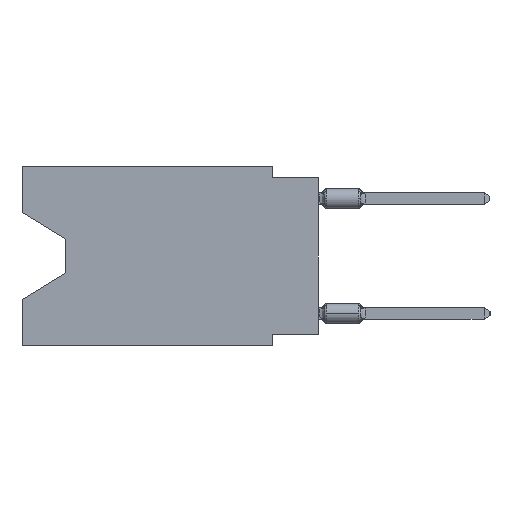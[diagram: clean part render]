
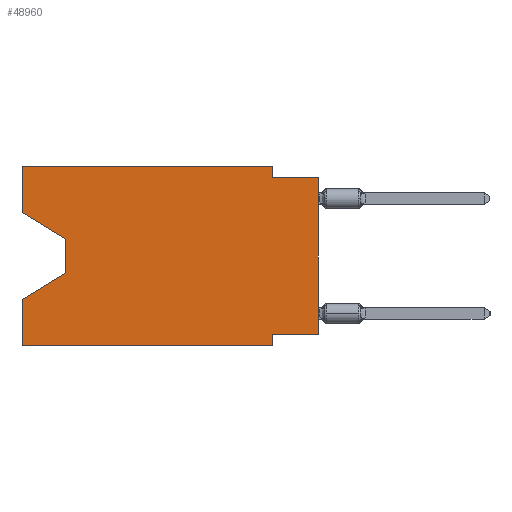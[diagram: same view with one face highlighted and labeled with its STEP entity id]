
A CAD part, left-side view. The second image highlights one B-rep face of the part: STEP entity #48960.
In plain terms, the highlighted planar face has unit normal (-1, 0, 0).
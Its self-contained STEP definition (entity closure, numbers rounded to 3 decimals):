
#575 = VECTOR ( 'NONE', #50226, 1000. ) ;
#576 = VERTEX_POINT ( 'NONE', #13247 ) ;
#620 = VERTEX_POINT ( 'NONE', #48480 ) ;
#1312 = CARTESIAN_POINT ( 'NONE',  ( 0., 16.383, -7.36 ) ) ;
#1710 = DIRECTION ( 'NONE',  ( 0., 0., 1. ) ) ;
#1779 = DIRECTION ( 'NONE',  ( 0., -1., 0. ) ) ;
#1916 = CARTESIAN_POINT ( 'NONE',  ( 0., 0., -9.271 ) ) ;
#2297 = VECTOR ( 'NONE', #49415, 1000. ) ;
#3335 = DIRECTION ( 'NONE',  ( 1., 0., 0. ) ) ;
#3434 = CARTESIAN_POINT ( 'NONE',  ( 0., 2.54, -9.271 ) ) ;
#3937 = VECTOR ( 'NONE', #17194, 1000. ) ;
#4367 = LINE ( 'NONE', #24657, #35956 ) ;
#5278 = LINE ( 'NONE', #1916, #10896 ) ;
#5329 = CARTESIAN_POINT ( 'NONE',  ( 0., 0., 0. ) ) ;
#5869 = VECTOR ( 'NONE', #15963, 1000. ) ;
#6452 = EDGE_CURVE ( 'NONE', #14874, #36099, #7994, .T. ) ;
#6680 = AXIS2_PLACEMENT_3D ( 'NONE', #38553, #3335, #34704 ) ;
#7187 = ORIENTED_EDGE ( 'NONE', *, *, #25041, .T. ) ;
#7193 = FACE_OUTER_BOUND ( 'NONE', #26918, .T. ) ;
#7867 = EDGE_CURVE ( 'NONE', #576, #23049, #26137, .T. ) ;
#7994 = LINE ( 'NONE', #23940, #48690 ) ;
#8058 = VERTEX_POINT ( 'NONE', #33026 ) ;
#8123 = VERTEX_POINT ( 'NONE', #17079 ) ;
#8860 = VECTOR ( 'NONE', #33204, 1000. ) ;
#9005 = CARTESIAN_POINT ( 'NONE',  ( 0., 0., -0.635 ) ) ;
#9218 = VERTEX_POINT ( 'NONE', #23315 ) ;
#10319 = CARTESIAN_POINT ( 'NONE',  ( 0., 16.383, -2.546 ) ) ;
#10844 = VERTEX_POINT ( 'NONE', #23974 ) ;
#10896 = VECTOR ( 'NONE', #17587, 1000. ) ;
#11327 = VECTOR ( 'NONE', #1710, 1000. ) ;
#12181 = EDGE_CURVE ( 'NONE', #620, #14874, #5278, .T. ) ;
#12405 = ORIENTED_EDGE ( 'NONE', *, *, #7867, .T. ) ;
#12762 = LINE ( 'NONE', #5329, #11327 ) ;
#13247 = CARTESIAN_POINT ( 'NONE',  ( 0., 13.97, -5.893 ) ) ;
#13327 = VERTEX_POINT ( 'NONE', #14257 ) ;
#14103 = CARTESIAN_POINT ( 'NONE',  ( 0., 2.54, 0. ) ) ;
#14257 = CARTESIAN_POINT ( 'NONE',  ( 0., 16.383, -2.546 ) ) ;
#14874 = VERTEX_POINT ( 'NONE', #3434 ) ;
#15162 = EDGE_CURVE ( 'NONE', #8123, #9218, #22070, .T. ) ;
#15177 = EDGE_CURVE ( 'NONE', #36685, #8123, #37746, .T. ) ;
#15963 = DIRECTION ( 'NONE',  ( 0., 0., 1. ) ) ;
#16169 = DIRECTION ( 'NONE',  ( 0., 0., 1. ) ) ;
#17079 = CARTESIAN_POINT ( 'NONE',  ( 0., 2.54, 0. ) ) ;
#17194 = DIRECTION ( 'NONE',  ( 0., 0., -1. ) ) ;
#17587 = DIRECTION ( 'NONE',  ( 0., 1., 0. ) ) ;
#18285 = LINE ( 'NONE', #29873, #8860 ) ;
#18729 = VECTOR ( 'NONE', #1779, 1000. ) ;
#22070 = LINE ( 'NONE', #14103, #3937 ) ;
#22883 = PLANE ( 'NONE',  #6680 ) ;
#23049 = VERTEX_POINT ( 'NONE', #1312 ) ;
#23315 = CARTESIAN_POINT ( 'NONE',  ( 0., 2.54, -0.635 ) ) ;
#23940 = CARTESIAN_POINT ( 'NONE',  ( 0., 2.54, -9.906 ) ) ;
#23974 = CARTESIAN_POINT ( 'NONE',  ( 0., 0., -0.635 ) ) ;
#24017 = EDGE_CURVE ( 'NONE', #29567, #576, #26823, .T. ) ;
#24657 = CARTESIAN_POINT ( 'NONE',  ( 0., 16.383, 0. ) ) ;
#24695 = DIRECTION ( 'NONE',  ( 0., -1., 0. ) ) ;
#25041 = EDGE_CURVE ( 'NONE', #620, #10844, #12762, .T. ) ;
#25495 = LINE ( 'NONE', #10319, #2297 ) ;
#26137 = LINE ( 'NONE', #45444, #39809 ) ;
#26687 = EDGE_CURVE ( 'NONE', #13327, #29567, #25495, .T. ) ;
#26753 = EDGE_CURVE ( 'NONE', #8058, #36099, #18285, .T. ) ;
#26801 = LINE ( 'NONE', #39113, #5869 ) ;
#26823 = LINE ( 'NONE', #35271, #575 ) ;
#26918 = EDGE_LOOP ( 'NONE', ( #46523, #27111, #12405, #46515, #47564, #32868, #32604, #7187, #33219, #41091, #41325, #44333 ) ) ;
#27111 = ORIENTED_EDGE ( 'NONE', *, *, #24017, .T. ) ;
#29441 = EDGE_CURVE ( 'NONE', #9218, #10844, #47848, .T. ) ;
#29567 = VERTEX_POINT ( 'NONE', #33161 ) ;
#29873 = CARTESIAN_POINT ( 'NONE',  ( 0., 16.383, -9.906 ) ) ;
#32398 = DIRECTION ( 'NONE',  ( 0., 0., -1. ) ) ;
#32604 = ORIENTED_EDGE ( 'NONE', *, *, #12181, .F. ) ;
#32868 = ORIENTED_EDGE ( 'NONE', *, *, #6452, .F. ) ;
#32883 = CARTESIAN_POINT ( 'NONE',  ( 0., 16.383, 0. ) ) ;
#33026 = CARTESIAN_POINT ( 'NONE',  ( 0., 16.383, -9.906 ) ) ;
#33161 = CARTESIAN_POINT ( 'NONE',  ( 0., 13.97, -4.013 ) ) ;
#33204 = DIRECTION ( 'NONE',  ( 0., -1., 0. ) ) ;
#33219 = ORIENTED_EDGE ( 'NONE', *, *, #29441, .F. ) ;
#34704 = DIRECTION ( 'NONE',  ( 0., 0., -1. ) ) ;
#35271 = CARTESIAN_POINT ( 'NONE',  ( 0., 13.97, -4.013 ) ) ;
#35703 = CARTESIAN_POINT ( 'NONE',  ( 0., 16.383, 0. ) ) ;
#35956 = VECTOR ( 'NONE', #16169, 1000. ) ;
#36099 = VERTEX_POINT ( 'NONE', #50202 ) ;
#36685 = VERTEX_POINT ( 'NONE', #35703 ) ;
#37746 = LINE ( 'NONE', #32883, #18729 ) ;
#37965 = DIRECTION ( 'NONE',  ( 0., 0.855, -0.519 ) ) ;
#38553 = CARTESIAN_POINT ( 'NONE',  ( 0., 16.383, 0. ) ) ;
#39113 = CARTESIAN_POINT ( 'NONE',  ( 0., 16.383, 0. ) ) ;
#39809 = VECTOR ( 'NONE', #37965, 1000. ) ;
#41091 = ORIENTED_EDGE ( 'NONE', *, *, #15162, .F. ) ;
#41325 = ORIENTED_EDGE ( 'NONE', *, *, #15177, .F. ) ;
#43103 = EDGE_CURVE ( 'NONE', #13327, #36685, #4367, .T. ) ;
#44333 = ORIENTED_EDGE ( 'NONE', *, *, #43103, .F. ) ;
#45444 = CARTESIAN_POINT ( 'NONE',  ( 0., 13.97, -5.893 ) ) ;
#46515 = ORIENTED_EDGE ( 'NONE', *, *, #48563, .F. ) ;
#46523 = ORIENTED_EDGE ( 'NONE', *, *, #26687, .T. ) ;
#47564 = ORIENTED_EDGE ( 'NONE', *, *, #26753, .T. ) ;
#47848 = LINE ( 'NONE', #9005, #50687 ) ;
#48480 = CARTESIAN_POINT ( 'NONE',  ( 0., 0., -9.271 ) ) ;
#48563 = EDGE_CURVE ( 'NONE', #8058, #23049, #26801, .T. ) ;
#48690 = VECTOR ( 'NONE', #32398, 1000. ) ;
#48960 = ADVANCED_FACE ( 'NONE', ( #7193 ), #22883, .F. ) ;
#49415 = DIRECTION ( 'NONE',  ( 0., -0.855, -0.519 ) ) ;
#50202 = CARTESIAN_POINT ( 'NONE',  ( 0., 2.54, -9.906 ) ) ;
#50226 = DIRECTION ( 'NONE',  ( 0., 0., -1. ) ) ;
#50687 = VECTOR ( 'NONE', #24695, 1000. ) ;
